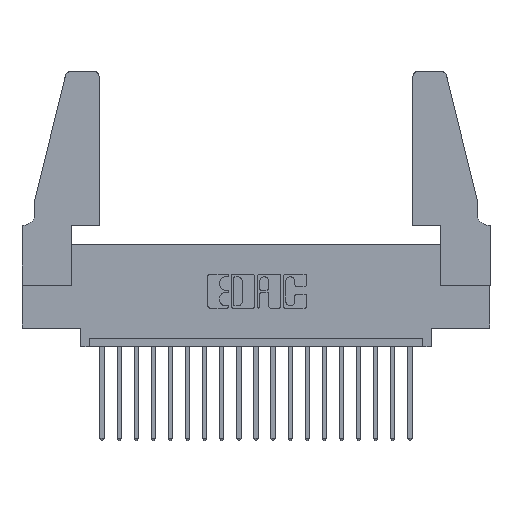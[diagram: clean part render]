
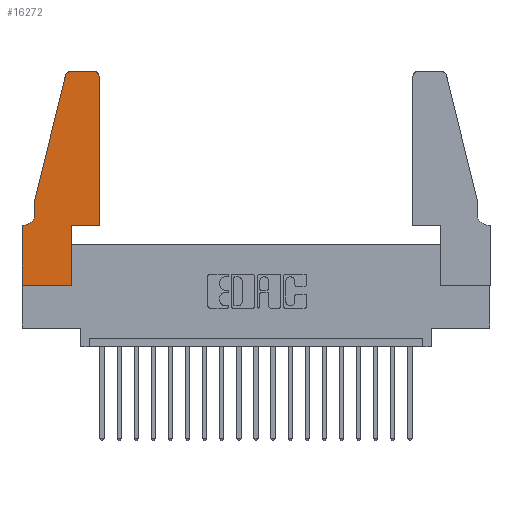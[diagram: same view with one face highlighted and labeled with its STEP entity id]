
A CAD part, top view. The second image highlights one B-rep face of the part: STEP entity #16272.
In plain terms, the highlighted planar face has unit normal (0, 0, 1).
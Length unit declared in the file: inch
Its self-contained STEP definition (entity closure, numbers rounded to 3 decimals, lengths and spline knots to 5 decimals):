
#283 = LINE ( 'NONE', #7962, #4081 ) ;
#1032 = EDGE_CURVE ( 'NONE', #19650, #12679, #14592, .T. ) ;
#1296 = ORIENTED_EDGE ( 'NONE', *, *, #10912, .T. ) ;
#1402 = DIRECTION ( 'NONE',  ( 1., 0., 0. ) ) ;
#1599 = VECTOR ( 'NONE', #1402, 39.37008 ) ;
#1773 = VECTOR ( 'NONE', #16087, 39.37008 ) ;
#1822 = EDGE_CURVE ( 'NONE', #12679, #3564, #3638, .T. ) ;
#1832 = VERTEX_POINT ( 'NONE', #15520 ) ;
#2053 = VECTOR ( 'NONE', #4245, 39.37008 ) ;
#2175 = CARTESIAN_POINT ( 'NONE',  ( 0.4505, 0.35, 0.37 ) ) ;
#2293 = DIRECTION ( 'NONE',  ( 0., -1., 0. ) ) ;
#2382 = EDGE_CURVE ( 'NONE', #17300, #11569, #283, .T. ) ;
#3108 = CARTESIAN_POINT ( 'NONE',  ( 0.284, 1.22, 0.37 ) ) ;
#3288 = CARTESIAN_POINT ( 'NONE',  ( 0.0755, 0.5, 0.37 ) ) ;
#3444 = LINE ( 'NONE', #6651, #7960 ) ;
#3546 = CARTESIAN_POINT ( 'NONE',  ( 0.2865, 0.35, 0.37 ) ) ;
#3564 = VERTEX_POINT ( 'NONE', #13390 ) ;
#3638 = LINE ( 'NONE', #3288, #11682 ) ;
#3842 = CARTESIAN_POINT ( 'NONE',  ( 0.4205, 1.22, 0.37 ) ) ;
#3980 = CARTESIAN_POINT ( 'NONE',  ( 0.4505, 0.35, 0.37 ) ) ;
#4081 = VECTOR ( 'NONE', #8024, 39.37008 ) ;
#4089 = CARTESIAN_POINT ( 'NONE',  ( 0.2605, 1.25, 0.37 ) ) ;
#4245 = DIRECTION ( 'NONE',  ( 1., 0., 0. ) ) ;
#4457 = EDGE_CURVE ( 'NONE', #1832, #19650, #17360, .T. ) ;
#4956 = VERTEX_POINT ( 'NONE', #19485 ) ;
#5465 = CIRCLE ( 'NONE', #18957, 0.03 ) ;
#5631 = LINE ( 'NONE', #2175, #1599 ) ;
#6161 = DIRECTION ( 'NONE',  ( 0., 0., 1. ) ) ;
#6211 = VERTEX_POINT ( 'NONE', #15357 ) ;
#6318 = AXIS2_PLACEMENT_3D ( 'NONE', #17082, #15619, #6496 ) ;
#6496 = DIRECTION ( 'NONE',  ( -1., 0., 0. ) ) ;
#6651 = CARTESIAN_POINT ( 'NONE',  ( 0.0755, 0.5, 0.37 ) ) ;
#6866 = ORIENTED_EDGE ( 'NONE', *, *, #1822, .T. ) ;
#6899 = DIRECTION ( 'NONE',  ( 0., 0., 1. ) ) ;
#7095 = FACE_OUTER_BOUND ( 'NONE', #19129, .T. ) ;
#7213 = CARTESIAN_POINT ( 'NONE',  ( 0., 0.35, 0.37 ) ) ;
#7532 = CARTESIAN_POINT ( 'NONE',  ( 0.2865, 0.35, 0.37 ) ) ;
#7713 = LINE ( 'NONE', #3980, #1773 ) ;
#7960 = VECTOR ( 'NONE', #14403, 39.37008 ) ;
#7962 = CARTESIAN_POINT ( 'NONE',  ( 0.0755, 0.35, 0.37 ) ) ;
#8024 = DIRECTION ( 'NONE',  ( -1., 0., 0. ) ) ;
#8033 = PLANE ( 'NONE',  #15661 ) ;
#8280 = EDGE_CURVE ( 'NONE', #15011, #14626, #12397, .T. ) ;
#8387 = VECTOR ( 'NONE', #14293, 39.37008 ) ;
#9080 = AXIS2_PLACEMENT_3D ( 'NONE', #3108, #6161, #9274 ) ;
#9256 = CARTESIAN_POINT ( 'NONE',  ( 0.284, 1.25, 0.37 ) ) ;
#9274 = DIRECTION ( 'NONE',  ( 1., 0., 0. ) ) ;
#9673 = DIRECTION ( 'NONE',  ( 1., 0., 0. ) ) ;
#9720 = CARTESIAN_POINT ( 'NONE',  ( 0., 0., 0.37 ) ) ;
#9794 = CARTESIAN_POINT ( 'NONE',  ( 0.4505, 0.35, 0.37 ) ) ;
#9938 = VECTOR ( 'NONE', #16450, 39.37008 ) ;
#9956 = ORIENTED_EDGE ( 'NONE', *, *, #17794, .T. ) ;
#10912 = EDGE_CURVE ( 'NONE', #14626, #14941, #5631, .T. ) ;
#11136 = DIRECTION ( 'NONE',  ( 0., 0., 1. ) ) ;
#11182 = LINE ( 'NONE', #9720, #16419 ) ;
#11569 = VERTEX_POINT ( 'NONE', #7213 ) ;
#11682 = VECTOR ( 'NONE', #18533, 39.37008 ) ;
#11715 = ORIENTED_EDGE ( 'NONE', *, *, #1032, .T. ) ;
#12153 = CARTESIAN_POINT ( 'NONE',  ( 0.2865, 0., 0.37 ) ) ;
#12397 = LINE ( 'NONE', #3546, #8387 ) ;
#12679 = VERTEX_POINT ( 'NONE', #16348 ) ;
#12689 = ORIENTED_EDGE ( 'NONE', *, *, #8280, .T. ) ;
#13190 = LINE ( 'NONE', #13314, #2053 ) ;
#13314 = CARTESIAN_POINT ( 'NONE',  ( 0., 0., 0.37 ) ) ;
#13390 = CARTESIAN_POINT ( 'NONE',  ( 0.0755, 0.5, 0.37 ) ) ;
#13622 = CARTESIAN_POINT ( 'NONE',  ( 0.0055, 0.35, 0.37 ) ) ;
#14293 = DIRECTION ( 'NONE',  ( 0., 1., 0. ) ) ;
#14334 = ORIENTED_EDGE ( 'NONE', *, *, #14758, .T. ) ;
#14348 = EDGE_CURVE ( 'NONE', #11569, #6211, #11182, .T. ) ;
#14403 = DIRECTION ( 'NONE',  ( 0., -1., 0. ) ) ;
#14592 = CIRCLE ( 'NONE', #9080, 0.03 ) ;
#14626 = VERTEX_POINT ( 'NONE', #7532 ) ;
#14758 = EDGE_CURVE ( 'NONE', #4956, #17300, #18341, .T. ) ;
#14842 = EDGE_CURVE ( 'NONE', #15791, #1832, #5465, .T. ) ;
#14941 = VERTEX_POINT ( 'NONE', #9794 ) ;
#15011 = VERTEX_POINT ( 'NONE', #12153 ) ;
#15312 = CARTESIAN_POINT ( 'NONE',  ( 0.4505, 1.22, 0.37 ) ) ;
#15357 = CARTESIAN_POINT ( 'NONE',  ( 0., 0., 0.37 ) ) ;
#15520 = CARTESIAN_POINT ( 'NONE',  ( 0.4205, 1.25, 0.37 ) ) ;
#15562 = ORIENTED_EDGE ( 'NONE', *, *, #18389, .T. ) ;
#15575 = ORIENTED_EDGE ( 'NONE', *, *, #2382, .T. ) ;
#15619 = DIRECTION ( 'NONE',  ( 0., 0., -1. ) ) ;
#15661 = AXIS2_PLACEMENT_3D ( 'NONE', #18686, #11136, #9673 ) ;
#15791 = VERTEX_POINT ( 'NONE', #15312 ) ;
#16087 = DIRECTION ( 'NONE',  ( 0., 1., 0. ) ) ;
#16272 = ADVANCED_FACE ( 'NONE', ( #7095 ), #8033, .T. ) ;
#16348 = CARTESIAN_POINT ( 'NONE',  ( 0.25487, 1.22718, 0.37 ) ) ;
#16419 = VECTOR ( 'NONE', #2293, 39.37008 ) ;
#16450 = DIRECTION ( 'NONE',  ( -1., 0., 0. ) ) ;
#17051 = ORIENTED_EDGE ( 'NONE', *, *, #14348, .T. ) ;
#17078 = ORIENTED_EDGE ( 'NONE', *, *, #4457, .T. ) ;
#17082 = CARTESIAN_POINT ( 'NONE',  ( 0.0055, 0.42, 0.37 ) ) ;
#17300 = VERTEX_POINT ( 'NONE', #13622 ) ;
#17360 = LINE ( 'NONE', #4089, #9938 ) ;
#17549 = DIRECTION ( 'NONE',  ( 1., 0., 0. ) ) ;
#17794 = EDGE_CURVE ( 'NONE', #6211, #15011, #13190, .T. ) ;
#18341 = CIRCLE ( 'NONE', #6318, 0.07 ) ;
#18389 = EDGE_CURVE ( 'NONE', #3564, #4956, #3444, .T. ) ;
#18390 = ORIENTED_EDGE ( 'NONE', *, *, #14842, .T. ) ;
#18516 = ORIENTED_EDGE ( 'NONE', *, *, #18664, .T. ) ;
#18533 = DIRECTION ( 'NONE',  ( -0.239, -0.971, 0. ) ) ;
#18664 = EDGE_CURVE ( 'NONE', #14941, #15791, #7713, .T. ) ;
#18686 = CARTESIAN_POINT ( 'NONE',  ( 0., 0.35, 0.37 ) ) ;
#18957 = AXIS2_PLACEMENT_3D ( 'NONE', #3842, #6899, #17549 ) ;
#19129 = EDGE_LOOP ( 'NONE', ( #17078, #11715, #6866, #15562, #14334, #15575, #17051, #9956, #12689, #1296, #18516, #18390 ) ) ;
#19485 = CARTESIAN_POINT ( 'NONE',  ( 0.0755, 0.42, 0.37 ) ) ;
#19650 = VERTEX_POINT ( 'NONE', #9256 ) ;
